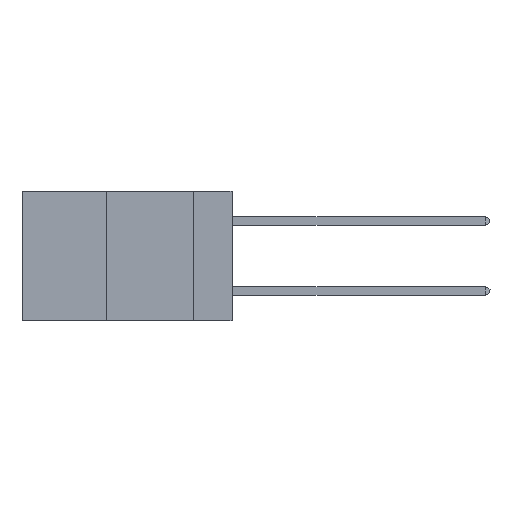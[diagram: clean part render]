
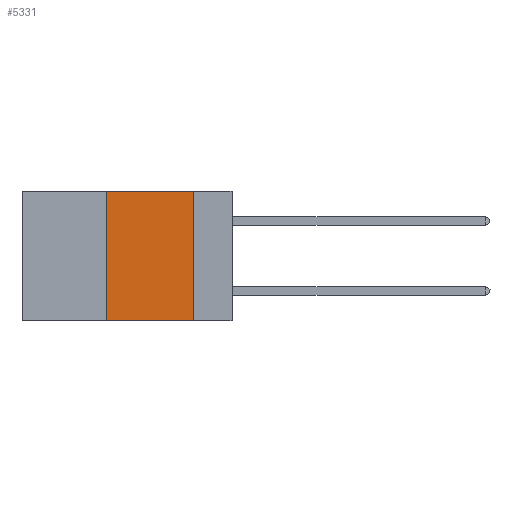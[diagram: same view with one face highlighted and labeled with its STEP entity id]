
A CAD part, left-side view. The second image highlights one B-rep face of the part: STEP entity #5331.
In plain terms, the highlighted planar face has unit normal (-1, 0, 0).
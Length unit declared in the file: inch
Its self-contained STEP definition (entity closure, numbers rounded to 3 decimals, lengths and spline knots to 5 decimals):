
#352 = EDGE_CURVE ( 'NONE', #7516, #867, #6125, .T. ) ;
#688 = AXIS2_PLACEMENT_3D ( 'NONE', #10104, #4210, #3294 ) ;
#867 = VERTEX_POINT ( 'NONE', #10048 ) ;
#1020 = DIRECTION ( 'NONE',  ( 0., 0., -1. ) ) ;
#2185 = CARTESIAN_POINT ( 'NONE',  ( 0., 0.36, 0. ) ) ;
#3089 = DIRECTION ( 'NONE',  ( 0., -1., 0. ) ) ;
#3158 = LINE ( 'NONE', #8035, #11067 ) ;
#3294 = DIRECTION ( 'NONE',  ( 0., 0., -1. ) ) ;
#4146 = FACE_OUTER_BOUND ( 'NONE', #12363, .T. ) ;
#4210 = DIRECTION ( 'NONE',  ( 1., 0., 0. ) ) ;
#4313 = ORIENTED_EDGE ( 'NONE', *, *, #8112, .T. ) ;
#4533 = EDGE_CURVE ( 'NONE', #9708, #7516, #7403, .T. ) ;
#4788 = VECTOR ( 'NONE', #12581, 39.37008 ) ;
#4986 = CARTESIAN_POINT ( 'NONE',  ( 0., 0.11, 0. ) ) ;
#5331 = ADVANCED_FACE ( 'NONE', ( #4146 ), #9236, .F. ) ;
#5693 = CARTESIAN_POINT ( 'NONE',  ( 0., 0.11, 0. ) ) ;
#5810 = VERTEX_POINT ( 'NONE', #7862 ) ;
#6125 = LINE ( 'NONE', #4986, #7188 ) ;
#6581 = CARTESIAN_POINT ( 'NONE',  ( 0., 0.36, 0. ) ) ;
#7175 = EDGE_CURVE ( 'NONE', #5810, #9708, #10907, .T. ) ;
#7188 = VECTOR ( 'NONE', #1020, 39.37008 ) ;
#7403 = LINE ( 'NONE', #9607, #4788 ) ;
#7516 = VERTEX_POINT ( 'NONE', #5693 ) ;
#7820 = ORIENTED_EDGE ( 'NONE', *, *, #4533, .F. ) ;
#7862 = CARTESIAN_POINT ( 'NONE',  ( 0., 0.36, -0.37 ) ) ;
#8035 = CARTESIAN_POINT ( 'NONE',  ( 0., 0.6, -0.37 ) ) ;
#8112 = EDGE_CURVE ( 'NONE', #5810, #867, #3158, .T. ) ;
#8655 = ORIENTED_EDGE ( 'NONE', *, *, #7175, .F. ) ;
#9236 = PLANE ( 'NONE',  #688 ) ;
#9510 = DIRECTION ( 'NONE',  ( 0., 0., 1. ) ) ;
#9607 = CARTESIAN_POINT ( 'NONE',  ( 0., 0.6, 0. ) ) ;
#9708 = VERTEX_POINT ( 'NONE', #2185 ) ;
#10048 = CARTESIAN_POINT ( 'NONE',  ( 0., 0.11, -0.37 ) ) ;
#10104 = CARTESIAN_POINT ( 'NONE',  ( 0., 0.6, 0. ) ) ;
#10294 = VECTOR ( 'NONE', #9510, 39.37008 ) ;
#10907 = LINE ( 'NONE', #6581, #10294 ) ;
#11067 = VECTOR ( 'NONE', #3089, 39.37008 ) ;
#11244 = ORIENTED_EDGE ( 'NONE', *, *, #352, .F. ) ;
#12363 = EDGE_LOOP ( 'NONE', ( #11244, #7820, #8655, #4313 ) ) ;
#12581 = DIRECTION ( 'NONE',  ( 0., -1., 0. ) ) ;
